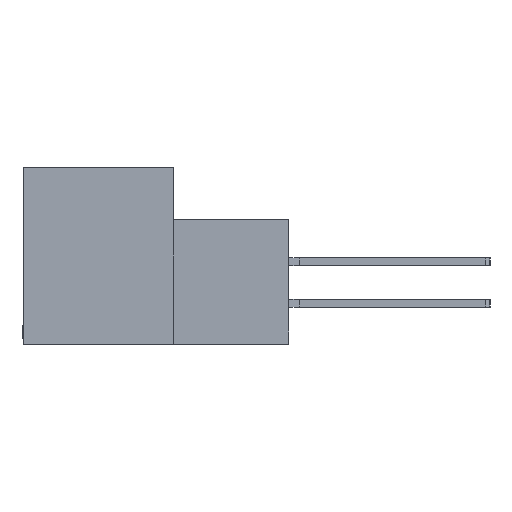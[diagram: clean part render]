
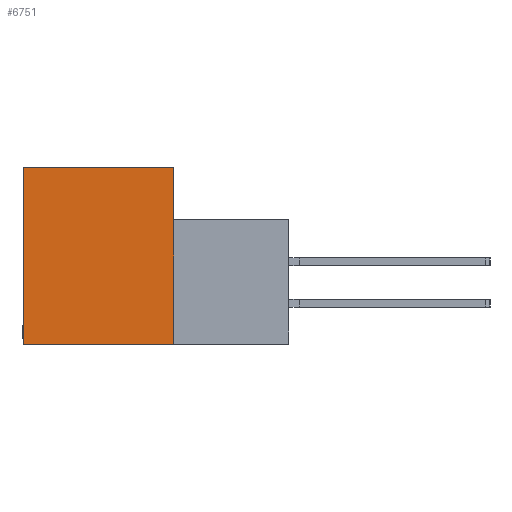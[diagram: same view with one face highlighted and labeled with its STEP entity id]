
A CAD part, left-side view. The second image highlights one B-rep face of the part: STEP entity #6751.
In plain terms, the highlighted planar face has unit normal (-1, 0, 0).
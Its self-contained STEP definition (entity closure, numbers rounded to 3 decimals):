
#544 = DIRECTION ( 'NONE',  ( 0., 0., -1. ) ) ;
#591 = CARTESIAN_POINT ( 'NONE',  ( 0., 11.506, 0. ) ) ;
#1385 = CARTESIAN_POINT ( 'NONE',  ( 0., 11.506, -13.487 ) ) ;
#1854 = DIRECTION ( 'NONE',  ( 1., 0., 0. ) ) ;
#4791 = DIRECTION ( 'NONE',  ( 0., 1., 0. ) ) ;
#4838 = VECTOR ( 'NONE', #15942, 1000. ) ;
#6751 = ADVANCED_FACE ( 'NONE', ( #31590 ), #32947, .F. ) ;
#8205 = EDGE_CURVE ( 'NONE', #27926, #20455, #39271, .T. ) ;
#9719 = VERTEX_POINT ( 'NONE', #16263 ) ;
#11578 = ORIENTED_EDGE ( 'NONE', *, *, #18403, .F. ) ;
#15541 = DIRECTION ( 'NONE',  ( 0., 0., 1. ) ) ;
#15751 = ORIENTED_EDGE ( 'NONE', *, *, #20584, .F. ) ;
#15897 = CARTESIAN_POINT ( 'NONE',  ( 0., 0., 0. ) ) ;
#15942 = DIRECTION ( 'NONE',  ( 0., -1., 0. ) ) ;
#16263 = CARTESIAN_POINT ( 'NONE',  ( 0., 0., 0. ) ) ;
#17497 = DIRECTION ( 'NONE',  ( 0., 0., -1. ) ) ;
#18403 = EDGE_CURVE ( 'NONE', #20455, #9719, #31052, .T. ) ;
#18413 = CARTESIAN_POINT ( 'NONE',  ( 0., 11.506, -13.487 ) ) ;
#20455 = VERTEX_POINT ( 'NONE', #591 ) ;
#20584 = EDGE_CURVE ( 'NONE', #31586, #27926, #36210, .T. ) ;
#23705 = VECTOR ( 'NONE', #15541, 1000. ) ;
#23960 = CARTESIAN_POINT ( 'NONE',  ( 0., 0., 0. ) ) ;
#25253 = LINE ( 'NONE', #15897, #35443 ) ;
#26495 = CARTESIAN_POINT ( 'NONE',  ( 0., -8.814, -13.487 ) ) ;
#26866 = ORIENTED_EDGE ( 'NONE', *, *, #38569, .F. ) ;
#27587 = AXIS2_PLACEMENT_3D ( 'NONE', #23960, #1854, #17497 ) ;
#27904 = ORIENTED_EDGE ( 'NONE', *, *, #8205, .F. ) ;
#27926 = VERTEX_POINT ( 'NONE', #1385 ) ;
#31052 = LINE ( 'NONE', #34556, #4838 ) ;
#31340 = VECTOR ( 'NONE', #4791, 1000. ) ;
#31586 = VERTEX_POINT ( 'NONE', #38264 ) ;
#31590 = FACE_OUTER_BOUND ( 'NONE', #35999, .T. ) ;
#32947 = PLANE ( 'NONE',  #27587 ) ;
#34556 = CARTESIAN_POINT ( 'NONE',  ( 0., 11.506, 0. ) ) ;
#35443 = VECTOR ( 'NONE', #544, 1000. ) ;
#35999 = EDGE_LOOP ( 'NONE', ( #15751, #26866, #11578, #27904 ) ) ;
#36210 = LINE ( 'NONE', #26495, #31340 ) ;
#38264 = CARTESIAN_POINT ( 'NONE',  ( 0., 0., -13.487 ) ) ;
#38569 = EDGE_CURVE ( 'NONE', #9719, #31586, #25253, .T. ) ;
#39271 = LINE ( 'NONE', #18413, #23705 ) ;
